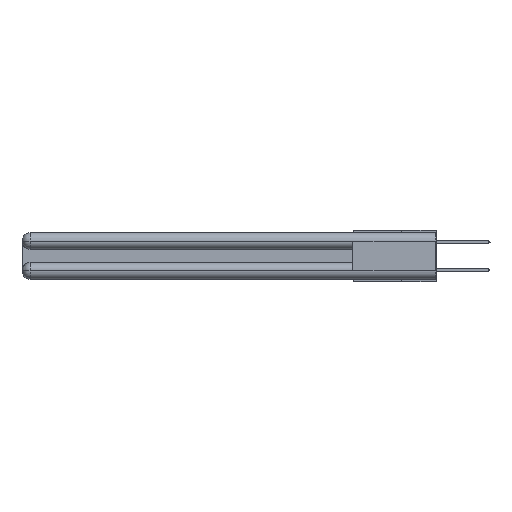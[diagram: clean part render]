
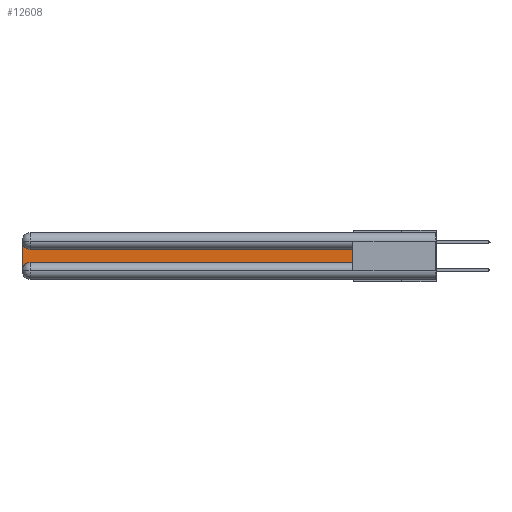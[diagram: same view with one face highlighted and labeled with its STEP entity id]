
A CAD part, left-side view. The second image highlights one B-rep face of the part: STEP entity #12608.
In plain terms, the highlighted planar face has unit normal (-1, 0, 0).
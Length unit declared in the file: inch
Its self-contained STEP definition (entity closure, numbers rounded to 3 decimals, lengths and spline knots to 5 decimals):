
#388 = EDGE_CURVE ( 'NONE', #7322, #22327, #29297, .T. ) ;
#874 = CARTESIAN_POINT ( 'NONE',  ( 0.075, 0.6, -0.2175 ) ) ;
#1224 = ORIENTED_EDGE ( 'NONE', *, *, #388, .T. ) ;
#1295 = ORIENTED_EDGE ( 'NONE', *, *, #5078, .T. ) ;
#3002 = CIRCLE ( 'NONE', #15794, 0.06 ) ;
#3663 = DIRECTION ( 'NONE',  ( 0., 1., 0. ) ) ;
#4044 = VERTEX_POINT ( 'NONE', #4103 ) ;
#4097 = LINE ( 'NONE', #874, #6940 ) ;
#4103 = CARTESIAN_POINT ( 'NONE',  ( 0.075, 0.6, -0.1225 ) ) ;
#4574 = DIRECTION ( 'NONE',  ( 1., 0., 0. ) ) ;
#4676 = PLANE ( 'NONE',  #4923 ) ;
#4923 = AXIS2_PLACEMENT_3D ( 'NONE', #8768, #4574, #25240 ) ;
#4973 = CARTESIAN_POINT ( 'NONE',  ( 0.075, 2.94, -0.2175 ) ) ;
#5078 = EDGE_CURVE ( 'NONE', #24433, #7322, #25491, .T. ) ;
#5584 = DIRECTION ( 'NONE',  ( 0., 0., 1. ) ) ;
#6066 = EDGE_CURVE ( 'NONE', #22327, #24861, #4097, .T. ) ;
#6487 = CARTESIAN_POINT ( 'NONE',  ( 0.075, 3., -0.2175 ) ) ;
#6865 = VECTOR ( 'NONE', #3663, 39.37008 ) ;
#6940 = VECTOR ( 'NONE', #7512, 39.37008 ) ;
#7322 = VERTEX_POINT ( 'NONE', #17318 ) ;
#7512 = DIRECTION ( 'NONE',  ( 0., -1., 0. ) ) ;
#8674 = DIRECTION ( 'NONE',  ( 0., 0., -1. ) ) ;
#8768 = CARTESIAN_POINT ( 'NONE',  ( 0.075, 3., -0.1225 ) ) ;
#10110 = ORIENTED_EDGE ( 'NONE', *, *, #21996, .T. ) ;
#10387 = AXIS2_PLACEMENT_3D ( 'NONE', #29102, #15419, #22438 ) ;
#10673 = LINE ( 'NONE', #28550, #21311 ) ;
#11490 = CARTESIAN_POINT ( 'NONE',  ( 0.075, 2.94, -0.1225 ) ) ;
#11945 = VERTEX_POINT ( 'NONE', #11490 ) ;
#12608 = ADVANCED_FACE ( 'NONE', ( #28237 ), #4676, .F. ) ;
#12914 = EDGE_CURVE ( 'NONE', #4044, #11945, #29252, .T. ) ;
#15114 = ORIENTED_EDGE ( 'NONE', *, *, #18365, .T. ) ;
#15185 = CARTESIAN_POINT ( 'NONE',  ( 0.075, 3., -0.0625 ) ) ;
#15419 = DIRECTION ( 'NONE',  ( 1., 0., 0. ) ) ;
#15794 = AXIS2_PLACEMENT_3D ( 'NONE', #19978, #27050, #8674 ) ;
#16176 = EDGE_LOOP ( 'NONE', ( #23984, #15114, #1295, #1224, #16381, #10110 ) ) ;
#16381 = ORIENTED_EDGE ( 'NONE', *, *, #6066, .T. ) ;
#17318 = CARTESIAN_POINT ( 'NONE',  ( 0.075, 3., -0.2775 ) ) ;
#18365 = EDGE_CURVE ( 'NONE', #11945, #24433, #3002, .T. ) ;
#19978 = CARTESIAN_POINT ( 'NONE',  ( 0.075, 2.94, -0.0625 ) ) ;
#21311 = VECTOR ( 'NONE', #5584, 39.37008 ) ;
#21996 = EDGE_CURVE ( 'NONE', #24861, #4044, #10673, .T. ) ;
#22279 = DIRECTION ( 'NONE',  ( 0., 0., -1. ) ) ;
#22327 = VERTEX_POINT ( 'NONE', #4973 ) ;
#22438 = DIRECTION ( 'NONE',  ( 0., 0., -1. ) ) ;
#23984 = ORIENTED_EDGE ( 'NONE', *, *, #12914, .T. ) ;
#24433 = VERTEX_POINT ( 'NONE', #15185 ) ;
#24861 = VERTEX_POINT ( 'NONE', #25368 ) ;
#25240 = DIRECTION ( 'NONE',  ( 0., 0., -1. ) ) ;
#25368 = CARTESIAN_POINT ( 'NONE',  ( 0.075, 0.6, -0.2175 ) ) ;
#25491 = LINE ( 'NONE', #6487, #26913 ) ;
#26221 = CARTESIAN_POINT ( 'NONE',  ( 0.075, 0.6, -0.1225 ) ) ;
#26913 = VECTOR ( 'NONE', #22279, 39.37008 ) ;
#27050 = DIRECTION ( 'NONE',  ( 1., 0., 0. ) ) ;
#28237 = FACE_OUTER_BOUND ( 'NONE', #16176, .T. ) ;
#28550 = CARTESIAN_POINT ( 'NONE',  ( 0.075, 0.6, -0.2175 ) ) ;
#29102 = CARTESIAN_POINT ( 'NONE',  ( 0.075, 2.94, -0.2775 ) ) ;
#29252 = LINE ( 'NONE', #26221, #6865 ) ;
#29297 = CIRCLE ( 'NONE', #10387, 0.06 ) ;
